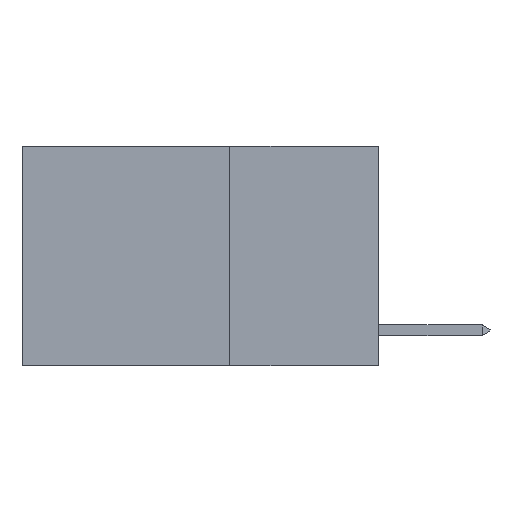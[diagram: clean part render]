
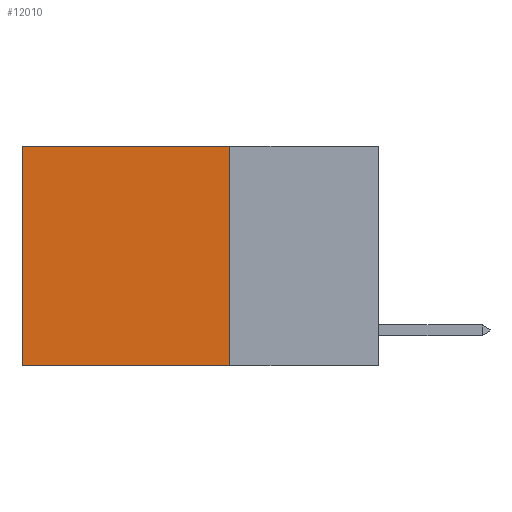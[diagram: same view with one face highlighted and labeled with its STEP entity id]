
A CAD part, left-side view. The second image highlights one B-rep face of the part: STEP entity #12010.
In plain terms, the highlighted planar face has unit normal (-1, 0, 0).
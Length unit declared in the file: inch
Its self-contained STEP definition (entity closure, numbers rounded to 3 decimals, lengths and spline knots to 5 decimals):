
#1511 = VERTEX_POINT ( 'NONE', #14077 ) ;
#1642 = VECTOR ( 'NONE', #24102, 39.37008 ) ;
#3295 = CARTESIAN_POINT ( 'NONE',  ( 0.2625, 0.25, 0. ) ) ;
#3571 = DIRECTION ( 'NONE',  ( 0., 1., 0. ) ) ;
#3911 = ORIENTED_EDGE ( 'NONE', *, *, #16263, .F. ) ;
#3957 = LINE ( 'NONE', #12764, #6190 ) ;
#4391 = VECTOR ( 'NONE', #9191, 39.37008 ) ;
#5506 = PLANE ( 'NONE',  #17257 ) ;
#6190 = VECTOR ( 'NONE', #3571, 39.37008 ) ;
#6565 = CARTESIAN_POINT ( 'NONE',  ( 0.2625, 0.25, 0. ) ) ;
#6613 = LINE ( 'NONE', #3295, #11749 ) ;
#7509 = EDGE_LOOP ( 'NONE', ( #15187, #21853, #3911, #14143 ) ) ;
#9191 = DIRECTION ( 'NONE',  ( 0., 0., -1. ) ) ;
#9433 = EDGE_CURVE ( 'NONE', #9839, #1511, #6613, .T. ) ;
#9839 = VERTEX_POINT ( 'NONE', #6565 ) ;
#11749 = VECTOR ( 'NONE', #28130, 39.37008 ) ;
#12010 = ADVANCED_FACE ( 'NONE', ( #23970 ), #5506, .F. ) ;
#12120 = DIRECTION ( 'NONE',  ( 0., 0., -1. ) ) ;
#12764 = CARTESIAN_POINT ( 'NONE',  ( 0.2625, 0.25, -0.37 ) ) ;
#13876 = VERTEX_POINT ( 'NONE', #28289 ) ;
#14077 = CARTESIAN_POINT ( 'NONE',  ( 0.2625, 0.6, 0. ) ) ;
#14143 = ORIENTED_EDGE ( 'NONE', *, *, #9433, .T. ) ;
#15187 = ORIENTED_EDGE ( 'NONE', *, *, #21916, .T. ) ;
#15230 = CARTESIAN_POINT ( 'NONE',  ( 0.2625, 0.25, -0.37 ) ) ;
#15258 = CARTESIAN_POINT ( 'NONE',  ( 0.2625, 0.6, 0. ) ) ;
#16263 = EDGE_CURVE ( 'NONE', #9839, #20368, #26611, .T. ) ;
#17257 = AXIS2_PLACEMENT_3D ( 'NONE', #20754, #20840, #12120 ) ;
#18204 = CARTESIAN_POINT ( 'NONE',  ( 0.2625, 0.25, 0. ) ) ;
#20368 = VERTEX_POINT ( 'NONE', #15230 ) ;
#20754 = CARTESIAN_POINT ( 'NONE',  ( 0.2625, 0.25, 0. ) ) ;
#20840 = DIRECTION ( 'NONE',  ( 1., 0., 0. ) ) ;
#21776 = EDGE_CURVE ( 'NONE', #20368, #13876, #3957, .T. ) ;
#21853 = ORIENTED_EDGE ( 'NONE', *, *, #21776, .F. ) ;
#21916 = EDGE_CURVE ( 'NONE', #1511, #13876, #25607, .T. ) ;
#23970 = FACE_OUTER_BOUND ( 'NONE', #7509, .T. ) ;
#24102 = DIRECTION ( 'NONE',  ( 0., 0., -1. ) ) ;
#25607 = LINE ( 'NONE', #15258, #1642 ) ;
#26611 = LINE ( 'NONE', #18204, #4391 ) ;
#28130 = DIRECTION ( 'NONE',  ( 0., 1., 0. ) ) ;
#28289 = CARTESIAN_POINT ( 'NONE',  ( 0.2625, 0.6, -0.37 ) ) ;
